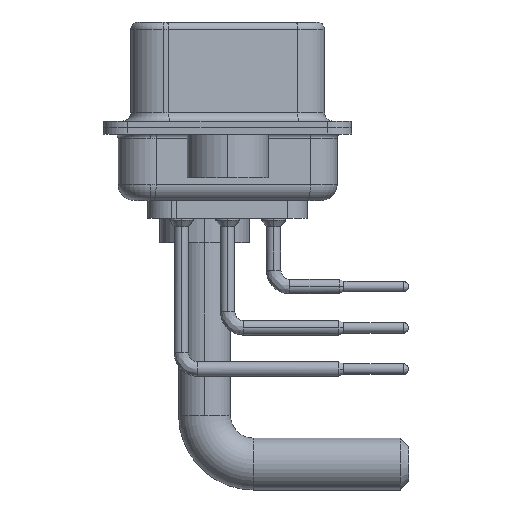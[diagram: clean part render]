
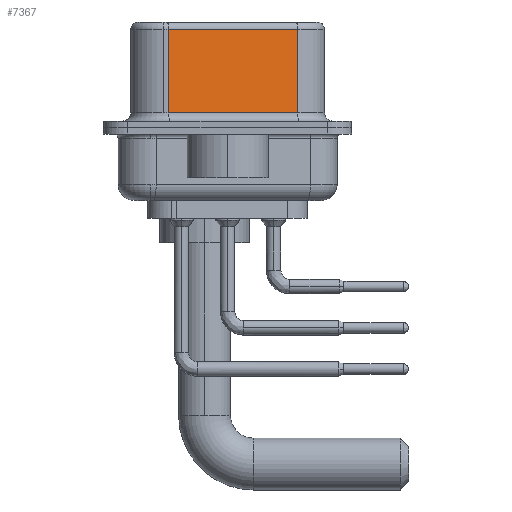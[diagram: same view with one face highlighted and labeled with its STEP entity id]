
A CAD part, left-side view. The second image highlights one B-rep face of the part: STEP entity #7367.
In plain terms, the highlighted planar face has unit normal (-0.985, -0.174, 0).
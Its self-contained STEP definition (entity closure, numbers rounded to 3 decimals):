
#81 = LINE ( 'NONE', #32076, #33644 ) ;
#965 = EDGE_CURVE ( 'NONE', #25572, #2364, #32838, .T. ) ;
#1249 = AXIS2_PLACEMENT_3D ( 'NONE', #2104, #4937, #2473 ) ;
#2104 = CARTESIAN_POINT ( 'NONE',  ( 5.132, -4.322, 6.52 ) ) ;
#2294 = VERTEX_POINT ( 'NONE', #8020 ) ;
#2358 = DIRECTION ( 'NONE',  ( 0., 0., -1. ) ) ;
#2364 = VERTEX_POINT ( 'NONE', #23383 ) ;
#2473 = DIRECTION ( 'NONE',  ( -0.174, 0.985, 0. ) ) ;
#2912 = CARTESIAN_POINT ( 'NONE',  ( 3.73, 3.628, 0.9 ) ) ;
#2923 = ORIENTED_EDGE ( 'NONE', *, *, #8921, .T. ) ;
#4937 = DIRECTION ( 'NONE',  ( 0.985, 0.174, 0. ) ) ;
#7188 = CARTESIAN_POINT ( 'NONE',  ( 3.73, 3.628, 6.52 ) ) ;
#7367 = ADVANCED_FACE ( 'NONE', ( #27681 ), #16710, .F. ) ;
#7855 = LINE ( 'NONE', #19422, #11801 ) ;
#8020 = CARTESIAN_POINT ( 'NONE',  ( 5.132, -4.322, 0.9 ) ) ;
#8921 = EDGE_CURVE ( 'NONE', #2364, #34935, #36164, .T. ) ;
#11801 = VECTOR ( 'NONE', #2358, 1000. ) ;
#13082 = ORIENTED_EDGE ( 'NONE', *, *, #32373, .T. ) ;
#14039 = ORIENTED_EDGE ( 'NONE', *, *, #965, .T. ) ;
#16710 = PLANE ( 'NONE',  #1249 ) ;
#16856 = VECTOR ( 'NONE', #30280, 1000. ) ;
#17943 = DIRECTION ( 'NONE',  ( -0.174, 0.985, 0. ) ) ;
#19422 = CARTESIAN_POINT ( 'NONE',  ( 5.132, -4.322, 6.52 ) ) ;
#19482 = VECTOR ( 'NONE', #17943, 1000. ) ;
#20365 = DIRECTION ( 'NONE',  ( 0.174, -0.985, 0. ) ) ;
#21143 = CARTESIAN_POINT ( 'NONE',  ( 5.132, -4.322, 6.02 ) ) ;
#22683 = ORIENTED_EDGE ( 'NONE', *, *, #30814, .F. ) ;
#23383 = CARTESIAN_POINT ( 'NONE',  ( 3.73, 3.628, 6.02 ) ) ;
#24153 = CARTESIAN_POINT ( 'NONE',  ( 5.132, -4.322, 6.02 ) ) ;
#24819 = EDGE_LOOP ( 'NONE', ( #22683, #14039, #2923, #13082 ) ) ;
#25572 = VERTEX_POINT ( 'NONE', #24153 ) ;
#27681 = FACE_OUTER_BOUND ( 'NONE', #24819, .T. ) ;
#30280 = DIRECTION ( 'NONE',  ( 0., 0., -1. ) ) ;
#30814 = EDGE_CURVE ( 'NONE', #25572, #2294, #7855, .T. ) ;
#32076 = CARTESIAN_POINT ( 'NONE',  ( 5.132, -4.322, 0.9 ) ) ;
#32373 = EDGE_CURVE ( 'NONE', #34935, #2294, #81, .T. ) ;
#32838 = LINE ( 'NONE', #21143, #19482 ) ;
#33644 = VECTOR ( 'NONE', #20365, 1000. ) ;
#34935 = VERTEX_POINT ( 'NONE', #2912 ) ;
#36164 = LINE ( 'NONE', #7188, #16856 ) ;
